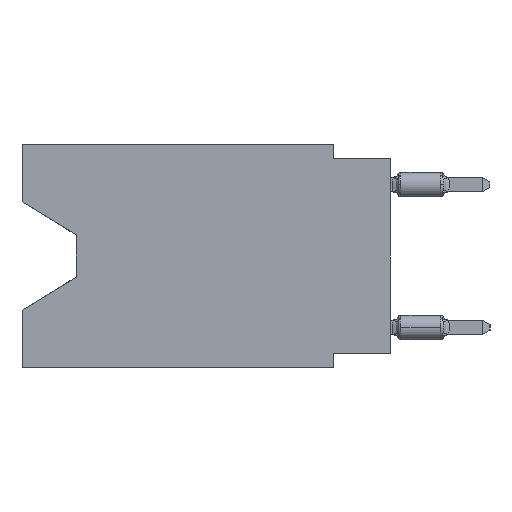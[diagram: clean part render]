
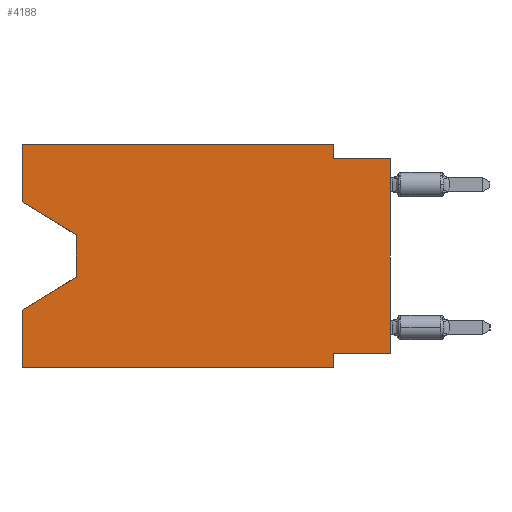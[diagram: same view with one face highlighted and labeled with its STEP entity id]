
A CAD part, left-side view. The second image highlights one B-rep face of the part: STEP entity #4188.
In plain terms, the highlighted planar face has unit normal (-1, 0, 0).
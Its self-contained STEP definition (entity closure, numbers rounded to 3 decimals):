
#245 = DIRECTION ( 'NONE',  ( 1., 0., 0. ) ) ;
#417 = CARTESIAN_POINT ( 'NONE',  ( 0., 16.383, -2.546 ) ) ;
#473 = VERTEX_POINT ( 'NONE', #11551 ) ;
#763 = ORIENTED_EDGE ( 'NONE', *, *, #7717, .F. ) ;
#1244 = VERTEX_POINT ( 'NONE', #5507 ) ;
#1964 = VERTEX_POINT ( 'NONE', #2630 ) ;
#2024 = LINE ( 'NONE', #11773, #16989 ) ;
#2197 = LINE ( 'NONE', #5778, #19977 ) ;
#2323 = DIRECTION ( 'NONE',  ( 0., 0., -1. ) ) ;
#2324 = LINE ( 'NONE', #17399, #21177 ) ;
#2630 = CARTESIAN_POINT ( 'NONE',  ( 0., 2.54, -9.271 ) ) ;
#2887 = CARTESIAN_POINT ( 'NONE',  ( 0., 13.97, -4.013 ) ) ;
#3387 = VERTEX_POINT ( 'NONE', #5207 ) ;
#3707 = CARTESIAN_POINT ( 'NONE',  ( 0., 16.383, 0. ) ) ;
#4049 = ORIENTED_EDGE ( 'NONE', *, *, #18952, .F. ) ;
#4188 = ADVANCED_FACE ( 'NONE', ( #15417 ), #14915, .F. ) ;
#4205 = VERTEX_POINT ( 'NONE', #5391 ) ;
#4316 = LINE ( 'NONE', #23568, #14892 ) ;
#4464 = AXIS2_PLACEMENT_3D ( 'NONE', #16893, #245, #19001 ) ;
#4478 = EDGE_CURVE ( 'NONE', #19084, #17594, #15531, .T. ) ;
#4597 = EDGE_CURVE ( 'NONE', #23085, #23594, #18131, .T. ) ;
#4886 = CARTESIAN_POINT ( 'NONE',  ( 0., 16.383, -9.906 ) ) ;
#5207 = CARTESIAN_POINT ( 'NONE',  ( 0., 2.54, -0.635 ) ) ;
#5391 = CARTESIAN_POINT ( 'NONE',  ( 0., 13.97, -5.893 ) ) ;
#5507 = CARTESIAN_POINT ( 'NONE',  ( 0., 2.54, -9.906 ) ) ;
#5778 = CARTESIAN_POINT ( 'NONE',  ( 0., 13.97, -4.013 ) ) ;
#5799 = ORIENTED_EDGE ( 'NONE', *, *, #23505, .T. ) ;
#5813 = DIRECTION ( 'NONE',  ( 0., -1., 0. ) ) ;
#6138 = DIRECTION ( 'NONE',  ( 0., 0., 1. ) ) ;
#6413 = ORIENTED_EDGE ( 'NONE', *, *, #4597, .F. ) ;
#6526 = ORIENTED_EDGE ( 'NONE', *, *, #4478, .T. ) ;
#6814 = DIRECTION ( 'NONE',  ( 0., -0.855, -0.519 ) ) ;
#7594 = DIRECTION ( 'NONE',  ( 0., 0.855, -0.519 ) ) ;
#7717 = EDGE_CURVE ( 'NONE', #7902, #473, #15051, .T. ) ;
#7902 = VERTEX_POINT ( 'NONE', #4886 ) ;
#8428 = VECTOR ( 'NONE', #14283, 1000. ) ;
#9143 = CARTESIAN_POINT ( 'NONE',  ( 0., 2.54, 0. ) ) ;
#9307 = EDGE_CURVE ( 'NONE', #4205, #473, #2024, .T. ) ;
#10211 = DIRECTION ( 'NONE',  ( 0., 0., -1. ) ) ;
#10216 = VECTOR ( 'NONE', #6814, 1000. ) ;
#11134 = VERTEX_POINT ( 'NONE', #9143 ) ;
#11339 = CARTESIAN_POINT ( 'NONE',  ( 0., 16.383, 0. ) ) ;
#11343 = EDGE_CURVE ( 'NONE', #3387, #17594, #17290, .T. ) ;
#11551 = CARTESIAN_POINT ( 'NONE',  ( 0., 16.383, -7.36 ) ) ;
#11773 = CARTESIAN_POINT ( 'NONE',  ( 0., 13.97, -5.893 ) ) ;
#12080 = CARTESIAN_POINT ( 'NONE',  ( 0., 16.383, 0. ) ) ;
#12302 = CARTESIAN_POINT ( 'NONE',  ( 0., 0., -0.635 ) ) ;
#13290 = CARTESIAN_POINT ( 'NONE',  ( 0., 0., -9.271 ) ) ;
#13469 = CARTESIAN_POINT ( 'NONE',  ( 0., 0., -0.635 ) ) ;
#13587 = VERTEX_POINT ( 'NONE', #2887 ) ;
#14152 = ORIENTED_EDGE ( 'NONE', *, *, #9307, .T. ) ;
#14163 = CARTESIAN_POINT ( 'NONE',  ( 0., 16.383, 0. ) ) ;
#14194 = EDGE_CURVE ( 'NONE', #13587, #4205, #2197, .T. ) ;
#14283 = DIRECTION ( 'NONE',  ( 0., 0., 1. ) ) ;
#14400 = VECTOR ( 'NONE', #24274, 1000. ) ;
#14598 = CARTESIAN_POINT ( 'NONE',  ( 0., 16.383, -2.546 ) ) ;
#14801 = ORIENTED_EDGE ( 'NONE', *, *, #11343, .F. ) ;
#14892 = VECTOR ( 'NONE', #15796, 1000. ) ;
#14915 = PLANE ( 'NONE',  #4464 ) ;
#15013 = LINE ( 'NONE', #13290, #14400 ) ;
#15051 = LINE ( 'NONE', #11339, #18542 ) ;
#15069 = EDGE_LOOP ( 'NONE', ( #16369, #23741, #14152, #763, #5799, #19173, #4049, #6526, #14801, #16170, #22206, #6413 ) ) ;
#15417 = FACE_OUTER_BOUND ( 'NONE', #15069, .T. ) ;
#15531 = LINE ( 'NONE', #23427, #15913 ) ;
#15796 = DIRECTION ( 'NONE',  ( 0., -1., 0. ) ) ;
#15913 = VECTOR ( 'NONE', #6138, 1000. ) ;
#16170 = ORIENTED_EDGE ( 'NONE', *, *, #19873, .F. ) ;
#16369 = ORIENTED_EDGE ( 'NONE', *, *, #22076, .T. ) ;
#16452 = EDGE_CURVE ( 'NONE', #1964, #1244, #17822, .T. ) ;
#16521 = VECTOR ( 'NONE', #5813, 1000. ) ;
#16893 = CARTESIAN_POINT ( 'NONE',  ( 0., 16.383, 0. ) ) ;
#16989 = VECTOR ( 'NONE', #7594, 1000. ) ;
#17290 = LINE ( 'NONE', #13469, #22466 ) ;
#17399 = CARTESIAN_POINT ( 'NONE',  ( 0., 2.54, 0. ) ) ;
#17594 = VERTEX_POINT ( 'NONE', #12302 ) ;
#17699 = CARTESIAN_POINT ( 'NONE',  ( 0., 2.54, -9.906 ) ) ;
#17822 = LINE ( 'NONE', #17699, #20837 ) ;
#18131 = LINE ( 'NONE', #14163, #8428 ) ;
#18542 = VECTOR ( 'NONE', #22596, 1000. ) ;
#18952 = EDGE_CURVE ( 'NONE', #19084, #1964, #15013, .T. ) ;
#19001 = DIRECTION ( 'NONE',  ( 0., 0., -1. ) ) ;
#19084 = VERTEX_POINT ( 'NONE', #23042 ) ;
#19173 = ORIENTED_EDGE ( 'NONE', *, *, #16452, .F. ) ;
#19873 = EDGE_CURVE ( 'NONE', #11134, #3387, #2324, .T. ) ;
#19977 = VECTOR ( 'NONE', #2323, 1000. ) ;
#20162 = LINE ( 'NONE', #14598, #10216 ) ;
#20837 = VECTOR ( 'NONE', #21768, 1000. ) ;
#21111 = DIRECTION ( 'NONE',  ( 0., -1., 0. ) ) ;
#21177 = VECTOR ( 'NONE', #10211, 1000. ) ;
#21768 = DIRECTION ( 'NONE',  ( 0., 0., -1. ) ) ;
#22076 = EDGE_CURVE ( 'NONE', #23085, #13587, #20162, .T. ) ;
#22190 = EDGE_CURVE ( 'NONE', #23594, #11134, #22751, .T. ) ;
#22206 = ORIENTED_EDGE ( 'NONE', *, *, #22190, .F. ) ;
#22466 = VECTOR ( 'NONE', #21111, 1000. ) ;
#22596 = DIRECTION ( 'NONE',  ( 0., 0., 1. ) ) ;
#22751 = LINE ( 'NONE', #3707, #16521 ) ;
#23042 = CARTESIAN_POINT ( 'NONE',  ( 0., 0., -9.271 ) ) ;
#23085 = VERTEX_POINT ( 'NONE', #417 ) ;
#23427 = CARTESIAN_POINT ( 'NONE',  ( 0., 0., 0. ) ) ;
#23505 = EDGE_CURVE ( 'NONE', #7902, #1244, #4316, .T. ) ;
#23568 = CARTESIAN_POINT ( 'NONE',  ( 0., 16.383, -9.906 ) ) ;
#23594 = VERTEX_POINT ( 'NONE', #12080 ) ;
#23741 = ORIENTED_EDGE ( 'NONE', *, *, #14194, .T. ) ;
#24274 = DIRECTION ( 'NONE',  ( 0., 1., 0. ) ) ;
